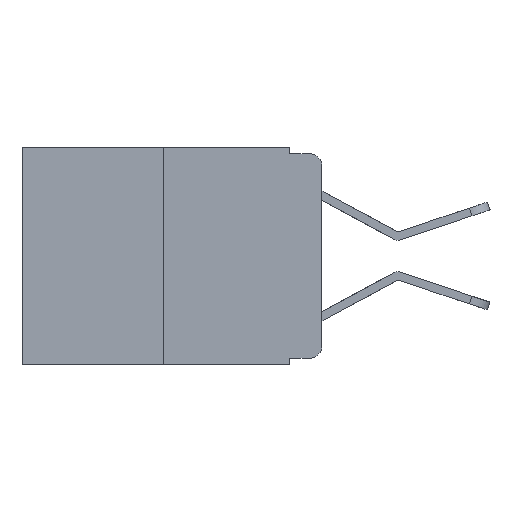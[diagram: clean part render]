
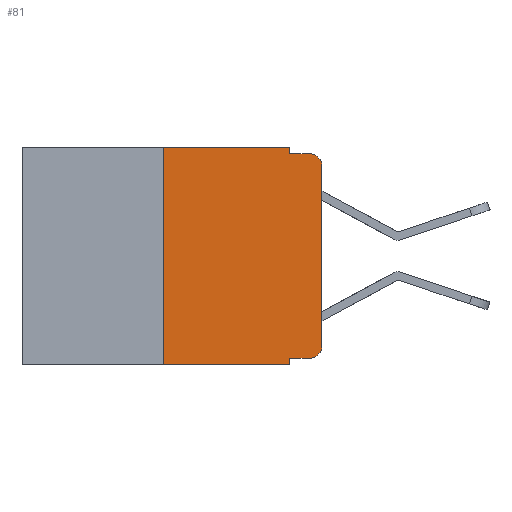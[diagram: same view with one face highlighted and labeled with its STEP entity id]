
A CAD part, left-side view. The second image highlights one B-rep face of the part: STEP entity #81.
In plain terms, the highlighted planar face has unit normal (-1, 0, 0).
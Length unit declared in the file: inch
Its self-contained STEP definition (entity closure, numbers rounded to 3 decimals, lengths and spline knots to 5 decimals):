
#19 = CARTESIAN_POINT ( 'NONE',  ( 0., 0.051, 0. ) ) ;
#80 = DIRECTION ( 'NONE',  ( 0., 0., 1. ) ) ;
#81 = ADVANCED_FACE ( 'NONE', ( #2442 ), #3964, .F. ) ;
#91 = EDGE_CURVE ( 'NONE', #3037, #11798, #1143, .T. ) ;
#638 = VERTEX_POINT ( 'NONE', #14243 ) ;
#1039 = CARTESIAN_POINT ( 'NONE',  ( 0., 0.051, 0. ) ) ;
#1119 = EDGE_CURVE ( 'NONE', #11798, #11941, #13370, .T. ) ;
#1143 = LINE ( 'NONE', #19, #4471 ) ;
#1827 = DIRECTION ( 'NONE',  ( 0., -1., 0. ) ) ;
#2056 = CARTESIAN_POINT ( 'NONE',  ( 0., 0.473, -0.343 ) ) ;
#2070 = EDGE_CURVE ( 'NONE', #7721, #11941, #3499, .T. ) ;
#2329 = CARTESIAN_POINT ( 'NONE',  ( 0., 0.051, -0.01 ) ) ;
#2369 = VECTOR ( 'NONE', #1827, 39.37008 ) ;
#2431 = DIRECTION ( 'NONE',  ( 0., 0., -1. ) ) ;
#2441 = EDGE_CURVE ( 'NONE', #8733, #3037, #14008, .T. ) ;
#2442 = FACE_OUTER_BOUND ( 'NONE', #7115, .T. ) ;
#2460 = DIRECTION ( 'NONE',  ( -1., 0., 0. ) ) ;
#2490 = CARTESIAN_POINT ( 'NONE',  ( 0., 0.02, -0.01 ) ) ;
#2604 = EDGE_CURVE ( 'NONE', #6183, #6662, #11336, .T. ) ;
#2906 = EDGE_CURVE ( 'NONE', #10977, #7721, #4569, .T. ) ;
#3037 = VERTEX_POINT ( 'NONE', #8274 ) ;
#3499 = CIRCLE ( 'NONE', #6025, 0.02 ) ;
#3503 = LINE ( 'NONE', #11470, #9533 ) ;
#3522 = CARTESIAN_POINT ( 'NONE',  ( 0., 0., -0.313 ) ) ;
#3571 = ORIENTED_EDGE ( 'NONE', *, *, #2070, .T. ) ;
#3695 = DIRECTION ( 'NONE',  ( 0., -1., 0. ) ) ;
#3964 = PLANE ( 'NONE',  #4226 ) ;
#4226 = AXIS2_PLACEMENT_3D ( 'NONE', #12468, #8704, #12931 ) ;
#4471 = VECTOR ( 'NONE', #10010, 39.37008 ) ;
#4569 = LINE ( 'NONE', #11416, #7141 ) ;
#4601 = VECTOR ( 'NONE', #11993, 39.37008 ) ;
#4828 = DIRECTION ( 'NONE',  ( 0., -1., 0. ) ) ;
#4876 = ORIENTED_EDGE ( 'NONE', *, *, #2441, .F. ) ;
#5039 = CARTESIAN_POINT ( 'NONE',  ( 0., 0.473, 0. ) ) ;
#5249 = CARTESIAN_POINT ( 'NONE',  ( 0., 0.02, -0.03 ) ) ;
#5801 = VECTOR ( 'NONE', #80, 39.37008 ) ;
#5930 = ORIENTED_EDGE ( 'NONE', *, *, #12872, .T. ) ;
#6025 = AXIS2_PLACEMENT_3D ( 'NONE', #5249, #11117, #8346 ) ;
#6183 = VERTEX_POINT ( 'NONE', #13920 ) ;
#6662 = VERTEX_POINT ( 'NONE', #13527 ) ;
#7115 = EDGE_LOOP ( 'NONE', ( #13259, #3571, #10603, #13954, #4876, #9292, #10817, #7516, #5930, #10342 ) ) ;
#7141 = VECTOR ( 'NONE', #9147, 39.37008 ) ;
#7516 = ORIENTED_EDGE ( 'NONE', *, *, #13559, .F. ) ;
#7721 = VERTEX_POINT ( 'NONE', #8836 ) ;
#8108 = LINE ( 'NONE', #1039, #13203 ) ;
#8274 = CARTESIAN_POINT ( 'NONE',  ( 0., 0.051, 0. ) ) ;
#8346 = DIRECTION ( 'NONE',  ( 0., 0., -1. ) ) ;
#8704 = DIRECTION ( 'NONE',  ( 1., 0., 0. ) ) ;
#8733 = VERTEX_POINT ( 'NONE', #13390 ) ;
#8836 = CARTESIAN_POINT ( 'NONE',  ( 0., 0., -0.03 ) ) ;
#9147 = DIRECTION ( 'NONE',  ( 0., 0., 1. ) ) ;
#9281 = CARTESIAN_POINT ( 'NONE',  ( 0., 0.02, -0.313 ) ) ;
#9292 = ORIENTED_EDGE ( 'NONE', *, *, #14295, .F. ) ;
#9533 = VECTOR ( 'NONE', #4828, 39.37008 ) ;
#10010 = DIRECTION ( 'NONE',  ( 0., 0., -1. ) ) ;
#10342 = ORIENTED_EDGE ( 'NONE', *, *, #12172, .T. ) ;
#10352 = AXIS2_PLACEMENT_3D ( 'NONE', #9281, #2460, #10371 ) ;
#10371 = DIRECTION ( 'NONE',  ( 0., 0., -1. ) ) ;
#10603 = ORIENTED_EDGE ( 'NONE', *, *, #1119, .F. ) ;
#10817 = ORIENTED_EDGE ( 'NONE', *, *, #2604, .T. ) ;
#10841 = VECTOR ( 'NONE', #3695, 39.37008 ) ;
#10977 = VERTEX_POINT ( 'NONE', #3522 ) ;
#11117 = DIRECTION ( 'NONE',  ( -1., 0., 0. ) ) ;
#11336 = LINE ( 'NONE', #2056, #2369 ) ;
#11416 = CARTESIAN_POINT ( 'NONE',  ( 0., 0., 0. ) ) ;
#11470 = CARTESIAN_POINT ( 'NONE',  ( 0., 0.051, -0.333 ) ) ;
#11553 = CIRCLE ( 'NONE', #10352, 0.02 ) ;
#11798 = VERTEX_POINT ( 'NONE', #2329 ) ;
#11941 = VERTEX_POINT ( 'NONE', #2490 ) ;
#11993 = DIRECTION ( 'NONE',  ( 0., -1., 0. ) ) ;
#12172 = EDGE_CURVE ( 'NONE', #14589, #10977, #11553, .T. ) ;
#12468 = CARTESIAN_POINT ( 'NONE',  ( 0., 0.473, 0. ) ) ;
#12872 = EDGE_CURVE ( 'NONE', #638, #14589, #3503, .T. ) ;
#12931 = DIRECTION ( 'NONE',  ( 0., 0., -1. ) ) ;
#13203 = VECTOR ( 'NONE', #2431, 39.37008 ) ;
#13227 = CARTESIAN_POINT ( 'NONE',  ( 0., 0.02, -0.333 ) ) ;
#13259 = ORIENTED_EDGE ( 'NONE', *, *, #2906, .T. ) ;
#13370 = LINE ( 'NONE', #13797, #4601 ) ;
#13390 = CARTESIAN_POINT ( 'NONE',  ( 0., 0.25, 0. ) ) ;
#13527 = CARTESIAN_POINT ( 'NONE',  ( 0., 0.051, -0.343 ) ) ;
#13559 = EDGE_CURVE ( 'NONE', #638, #6662, #8108, .T. ) ;
#13797 = CARTESIAN_POINT ( 'NONE',  ( 0., 0.051, -0.01 ) ) ;
#13920 = CARTESIAN_POINT ( 'NONE',  ( 0., 0.25, -0.343 ) ) ;
#13921 = CARTESIAN_POINT ( 'NONE',  ( 0., 0.25, 0. ) ) ;
#13954 = ORIENTED_EDGE ( 'NONE', *, *, #91, .F. ) ;
#14008 = LINE ( 'NONE', #5039, #10841 ) ;
#14243 = CARTESIAN_POINT ( 'NONE',  ( 0., 0.051, -0.333 ) ) ;
#14295 = EDGE_CURVE ( 'NONE', #6183, #8733, #14820, .T. ) ;
#14589 = VERTEX_POINT ( 'NONE', #13227 ) ;
#14820 = LINE ( 'NONE', #13921, #5801 ) ;
